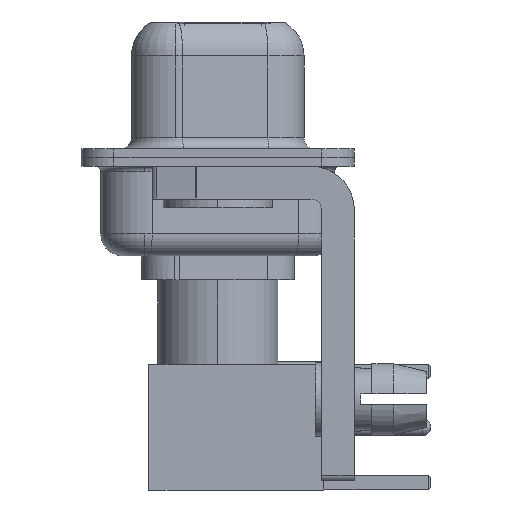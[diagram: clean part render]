
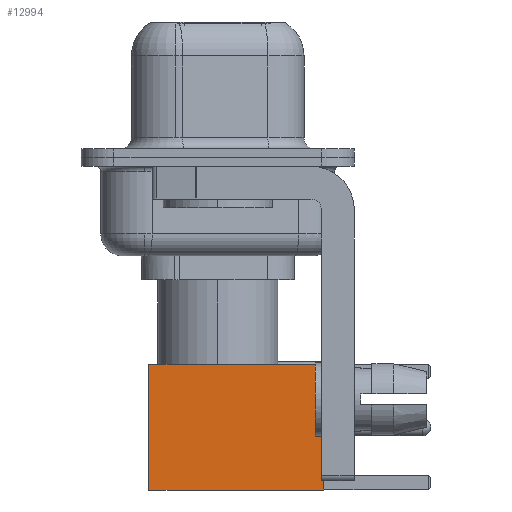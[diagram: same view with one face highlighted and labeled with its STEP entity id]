
A CAD part, left-side view. The second image highlights one B-rep face of the part: STEP entity #12994.
In plain terms, the highlighted face is planar.
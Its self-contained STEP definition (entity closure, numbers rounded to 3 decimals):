
#62 = CARTESIAN_POINT ( 'NONE',  ( 0., 2.875, 8. ) ) ;
#110 = CARTESIAN_POINT ( 'NONE',  ( 2.875, 2.875, 0. ) ) ;
#863 = DIRECTION ( 'NONE',  ( 0., 0., -1. ) ) ;
#1547 = LINE ( 'NONE', #62, #9784 ) ;
#2241 = LINE ( 'NONE', #5337, #20008 ) ;
#2460 = ORIENTED_EDGE ( 'NONE', *, *, #19774, .T. ) ;
#4935 = ORIENTED_EDGE ( 'NONE', *, *, #9588, .T. ) ;
#5168 = PLANE ( 'NONE',  #11355 ) ;
#5337 = CARTESIAN_POINT ( 'NONE',  ( 0., 2.875, 0. ) ) ;
#5864 = VERTEX_POINT ( 'NONE', #19300 ) ;
#6425 = VERTEX_POINT ( 'NONE', #21180 ) ;
#6635 = ORIENTED_EDGE ( 'NONE', *, *, #21102, .F. ) ;
#7345 = LINE ( 'NONE', #14339, #11574 ) ;
#7881 = CARTESIAN_POINT ( 'NONE',  ( 2.875, 2.875, 0. ) ) ;
#7929 = VECTOR ( 'NONE', #863, 1000. ) ;
#8510 = DIRECTION ( 'NONE',  ( 0., 0., 1. ) ) ;
#9125 = EDGE_CURVE ( 'NONE', #6425, #18819, #7345, .T. ) ;
#9588 = EDGE_CURVE ( 'NONE', #5864, #16451, #16598, .T. ) ;
#9784 = VECTOR ( 'NONE', #13961, 1000. ) ;
#11355 = AXIS2_PLACEMENT_3D ( 'NONE', #110, #21093, #8510 ) ;
#11574 = VECTOR ( 'NONE', #21312, 1000. ) ;
#12994 = ADVANCED_FACE ( 'NONE', ( #20983 ), #5168, .T. ) ;
#13961 = DIRECTION ( 'NONE',  ( -1., 0., 0. ) ) ;
#14339 = CARTESIAN_POINT ( 'NONE',  ( -2.875, 2.875, 0. ) ) ;
#16019 = DIRECTION ( 'NONE',  ( -1., 0., 0. ) ) ;
#16451 = VERTEX_POINT ( 'NONE', #20436 ) ;
#16598 = LINE ( 'NONE', #7881, #7929 ) ;
#16810 = CARTESIAN_POINT ( 'NONE',  ( -2.875, 2.875, 0. ) ) ;
#18599 = EDGE_LOOP ( 'NONE', ( #4935, #2460, #21723, #6635 ) ) ;
#18819 = VERTEX_POINT ( 'NONE', #16810 ) ;
#19300 = CARTESIAN_POINT ( 'NONE',  ( 2.875, 2.875, 8. ) ) ;
#19774 = EDGE_CURVE ( 'NONE', #16451, #18819, #2241, .T. ) ;
#20008 = VECTOR ( 'NONE', #16019, 1000. ) ;
#20436 = CARTESIAN_POINT ( 'NONE',  ( 2.875, 2.875, 0. ) ) ;
#20983 = FACE_OUTER_BOUND ( 'NONE', #18599, .T. ) ;
#21093 = DIRECTION ( 'NONE',  ( 0., 1., 0. ) ) ;
#21102 = EDGE_CURVE ( 'NONE', #5864, #6425, #1547, .T. ) ;
#21180 = CARTESIAN_POINT ( 'NONE',  ( -2.875, 2.875, 8. ) ) ;
#21312 = DIRECTION ( 'NONE',  ( 0., 0., -1. ) ) ;
#21723 = ORIENTED_EDGE ( 'NONE', *, *, #9125, .F. ) ;
